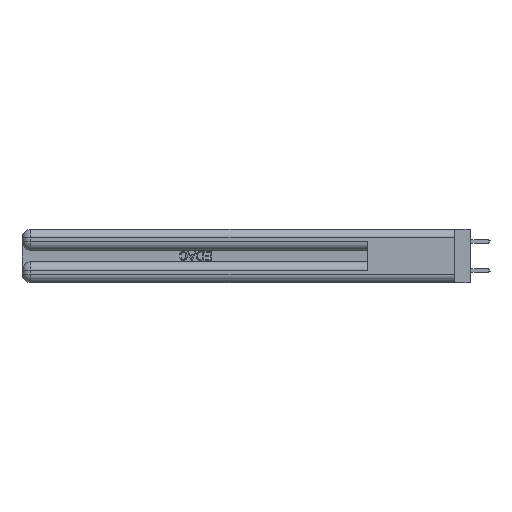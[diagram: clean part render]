
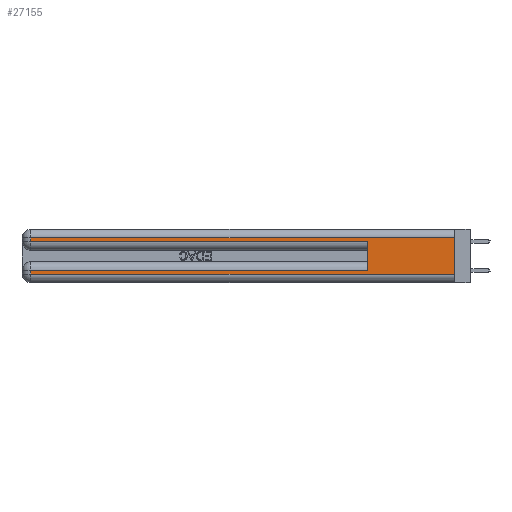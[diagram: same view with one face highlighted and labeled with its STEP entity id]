
A CAD part, left-side view. The second image highlights one B-rep face of the part: STEP entity #27155.
In plain terms, the highlighted planar face has unit normal (-1, 0, 0).
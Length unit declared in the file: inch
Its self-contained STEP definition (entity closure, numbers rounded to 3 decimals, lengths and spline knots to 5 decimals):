
#378 = CARTESIAN_POINT ( 'NONE',  ( 0., 0.6, 0.285 ) ) ;
#1120 = DIRECTION ( 'NONE',  ( 0., 0., -1. ) ) ;
#1175 = EDGE_CURVE ( 'NONE', #6993, #22458, #33616, .T. ) ;
#1842 = ORIENTED_EDGE ( 'NONE', *, *, #9871, .T. ) ;
#2862 = VECTOR ( 'NONE', #5204, 39.37008 ) ;
#3809 = VERTEX_POINT ( 'NONE', #29443 ) ;
#5093 = FACE_OUTER_BOUND ( 'NONE', #35389, .T. ) ;
#5204 = DIRECTION ( 'NONE',  ( 0., 0., -1. ) ) ;
#6296 = ORIENTED_EDGE ( 'NONE', *, *, #25011, .F. ) ;
#6993 = VERTEX_POINT ( 'NONE', #41995 ) ;
#7111 = VERTEX_POINT ( 'NONE', #24489 ) ;
#8304 = CARTESIAN_POINT ( 'NONE',  ( 0., 2.94, 0.37 ) ) ;
#9871 = EDGE_CURVE ( 'NONE', #3809, #12034, #35801, .T. ) ;
#11157 = CARTESIAN_POINT ( 'NONE',  ( 0., 0., 0.285 ) ) ;
#11641 = DIRECTION ( 'NONE',  ( 0., 0., -1. ) ) ;
#12034 = VERTEX_POINT ( 'NONE', #17598 ) ;
#13129 = CARTESIAN_POINT ( 'NONE',  ( 0., 0., 0.06 ) ) ;
#13724 = LINE ( 'NONE', #27871, #2862 ) ;
#14481 = DIRECTION ( 'NONE',  ( 0., -1., 0. ) ) ;
#15164 = ORIENTED_EDGE ( 'NONE', *, *, #35004, .T. ) ;
#17080 = VECTOR ( 'NONE', #42400, 39.37008 ) ;
#17598 = CARTESIAN_POINT ( 'NONE',  ( 0., 2.94, 0.31 ) ) ;
#17924 = LINE ( 'NONE', #11157, #32447 ) ;
#19134 = DIRECTION ( 'NONE',  ( 0., 0., -1. ) ) ;
#19254 = LINE ( 'NONE', #40801, #27030 ) ;
#19846 = DIRECTION ( 'NONE',  ( 0., 1., 0. ) ) ;
#21644 = EDGE_CURVE ( 'NONE', #24724, #24333, #17924, .T. ) ;
#22283 = CARTESIAN_POINT ( 'NONE',  ( 0., 2.94, 0.285 ) ) ;
#22458 = VERTEX_POINT ( 'NONE', #13129 ) ;
#22461 = DIRECTION ( 'NONE',  ( 1., 0., 0. ) ) ;
#22759 = PLANE ( 'NONE',  #38503 ) ;
#22797 = EDGE_CURVE ( 'NONE', #7111, #24333, #29330, .T. ) ;
#23301 = CARTESIAN_POINT ( 'NONE',  ( 0., 0., 0.06 ) ) ;
#23392 = ORIENTED_EDGE ( 'NONE', *, *, #30396, .T. ) ;
#24021 = ORIENTED_EDGE ( 'NONE', *, *, #24376, .T. ) ;
#24050 = CARTESIAN_POINT ( 'NONE',  ( 0., 0.6, 0.145 ) ) ;
#24333 = VERTEX_POINT ( 'NONE', #378 ) ;
#24376 = EDGE_CURVE ( 'NONE', #7111, #34526, #29708, .T. ) ;
#24489 = CARTESIAN_POINT ( 'NONE',  ( 0., 0.6, 0.085 ) ) ;
#24724 = VERTEX_POINT ( 'NONE', #22283 ) ;
#24921 = ORIENTED_EDGE ( 'NONE', *, *, #21644, .T. ) ;
#25011 = EDGE_CURVE ( 'NONE', #3809, #22458, #19254, .T. ) ;
#27030 = VECTOR ( 'NONE', #1120, 39.37008 ) ;
#27155 = ADVANCED_FACE ( 'NONE', ( #5093 ), #22759, .F. ) ;
#27197 = VECTOR ( 'NONE', #33679, 39.37008 ) ;
#27871 = CARTESIAN_POINT ( 'NONE',  ( 0., 2.94, 0.37 ) ) ;
#28516 = VECTOR ( 'NONE', #31787, 39.37008 ) ;
#28670 = VECTOR ( 'NONE', #19846, 39.37008 ) ;
#28703 = VECTOR ( 'NONE', #11641, 39.37008 ) ;
#29021 = CARTESIAN_POINT ( 'NONE',  ( 0., 0., 0.085 ) ) ;
#29229 = CARTESIAN_POINT ( 'NONE',  ( 0., 2.94, 0.085 ) ) ;
#29330 = LINE ( 'NONE', #24050, #27197 ) ;
#29443 = CARTESIAN_POINT ( 'NONE',  ( 0., 0., 0.31 ) ) ;
#29708 = LINE ( 'NONE', #29021, #28670 ) ;
#29742 = LINE ( 'NONE', #8304, #28703 ) ;
#30396 = EDGE_CURVE ( 'NONE', #12034, #24724, #29742, .T. ) ;
#31552 = CARTESIAN_POINT ( 'NONE',  ( 0., 0., 0.31 ) ) ;
#31787 = DIRECTION ( 'NONE',  ( 0., -1., 0. ) ) ;
#32447 = VECTOR ( 'NONE', #14481, 39.37008 ) ;
#33616 = LINE ( 'NONE', #23301, #28516 ) ;
#33679 = DIRECTION ( 'NONE',  ( 0., 0., 1. ) ) ;
#34526 = VERTEX_POINT ( 'NONE', #29229 ) ;
#35004 = EDGE_CURVE ( 'NONE', #34526, #6993, #13724, .T. ) ;
#35389 = EDGE_LOOP ( 'NONE', ( #6296, #1842, #23392, #24921, #39951, #24021, #15164, #39716 ) ) ;
#35439 = CARTESIAN_POINT ( 'NONE',  ( 0., 0., 0.37 ) ) ;
#35801 = LINE ( 'NONE', #31552, #17080 ) ;
#38503 = AXIS2_PLACEMENT_3D ( 'NONE', #35439, #22461, #19134 ) ;
#39716 = ORIENTED_EDGE ( 'NONE', *, *, #1175, .T. ) ;
#39951 = ORIENTED_EDGE ( 'NONE', *, *, #22797, .F. ) ;
#40801 = CARTESIAN_POINT ( 'NONE',  ( 0., 0., 0.37 ) ) ;
#41995 = CARTESIAN_POINT ( 'NONE',  ( 0., 2.94, 0.06 ) ) ;
#42400 = DIRECTION ( 'NONE',  ( 0., 1., 0. ) ) ;
